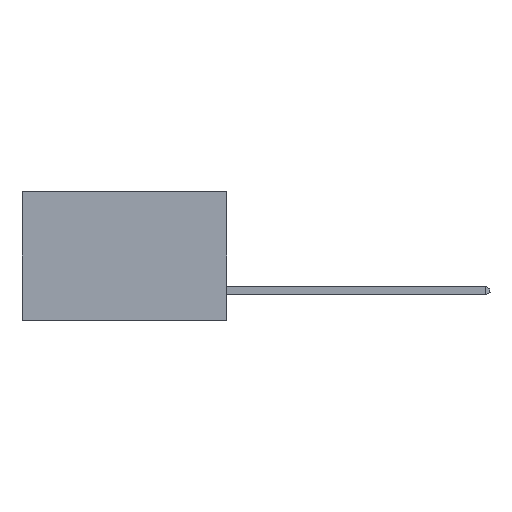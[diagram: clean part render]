
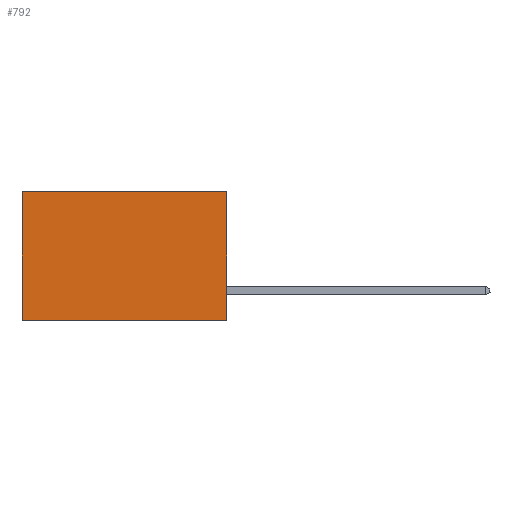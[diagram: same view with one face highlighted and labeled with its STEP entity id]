
A CAD part, left-side view. The second image highlights one B-rep face of the part: STEP entity #792.
In plain terms, the highlighted planar face has unit normal (-1, 0, 0).
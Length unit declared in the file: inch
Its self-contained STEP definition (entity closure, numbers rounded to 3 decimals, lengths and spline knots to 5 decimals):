
#745 = EDGE_CURVE ( 'NONE', #2251, #3498, #1872, .T. ) ;
#792 = ADVANCED_FACE ( 'NONE', ( #8173 ), #7313, .F. ) ;
#811 = VERTEX_POINT ( 'NONE', #3676 ) ;
#1142 = DIRECTION ( 'NONE',  ( 0., 0., -1. ) ) ;
#1163 = CARTESIAN_POINT ( 'NONE',  ( 0.277, 0., -0.37 ) ) ;
#1389 = LINE ( 'NONE', #1163, #8323 ) ;
#1849 = CARTESIAN_POINT ( 'NONE',  ( 0.277, 0., 0. ) ) ;
#1872 = LINE ( 'NONE', #6488, #7345 ) ;
#2251 = VERTEX_POINT ( 'NONE', #4747 ) ;
#2372 = DIRECTION ( 'NONE',  ( 0., 0., -1. ) ) ;
#3368 = DIRECTION ( 'NONE',  ( 0., 1., 0. ) ) ;
#3384 = CARTESIAN_POINT ( 'NONE',  ( 0.277, 0., -0.37 ) ) ;
#3392 = CARTESIAN_POINT ( 'NONE',  ( 0.277, 0., -0.37 ) ) ;
#3498 = VERTEX_POINT ( 'NONE', #4994 ) ;
#3511 = VECTOR ( 'NONE', #3368, 39.37008 ) ;
#3652 = ORIENTED_EDGE ( 'NONE', *, *, #745, .T. ) ;
#3676 = CARTESIAN_POINT ( 'NONE',  ( 0.277, 0., -0.37 ) ) ;
#3836 = EDGE_CURVE ( 'NONE', #811, #3498, #8687, .T. ) ;
#3866 = ORIENTED_EDGE ( 'NONE', *, *, #5896, .T. ) ;
#4086 = AXIS2_PLACEMENT_3D ( 'NONE', #3384, #6368, #6469 ) ;
#4171 = EDGE_CURVE ( 'NONE', #6514, #811, #1389, .T. ) ;
#4243 = EDGE_LOOP ( 'NONE', ( #3652, #5565, #7251, #3866 ) ) ;
#4747 = CARTESIAN_POINT ( 'NONE',  ( 0.277, 0.59, 0. ) ) ;
#4994 = CARTESIAN_POINT ( 'NONE',  ( 0.277, 0.59, -0.37 ) ) ;
#5565 = ORIENTED_EDGE ( 'NONE', *, *, #3836, .F. ) ;
#5896 = EDGE_CURVE ( 'NONE', #6514, #2251, #7583, .T. ) ;
#5906 = VECTOR ( 'NONE', #7559, 39.37008 ) ;
#6368 = DIRECTION ( 'NONE',  ( 1., 0., 0. ) ) ;
#6469 = DIRECTION ( 'NONE',  ( 0., 0., -1. ) ) ;
#6488 = CARTESIAN_POINT ( 'NONE',  ( 0.277, 0.59, -0.37 ) ) ;
#6514 = VERTEX_POINT ( 'NONE', #1849 ) ;
#6945 = CARTESIAN_POINT ( 'NONE',  ( 0.277, 0., 0. ) ) ;
#7251 = ORIENTED_EDGE ( 'NONE', *, *, #4171, .F. ) ;
#7313 = PLANE ( 'NONE',  #4086 ) ;
#7345 = VECTOR ( 'NONE', #2372, 39.37008 ) ;
#7559 = DIRECTION ( 'NONE',  ( 0., 1., 0. ) ) ;
#7583 = LINE ( 'NONE', #6945, #5906 ) ;
#8173 = FACE_OUTER_BOUND ( 'NONE', #4243, .T. ) ;
#8323 = VECTOR ( 'NONE', #1142, 39.37008 ) ;
#8687 = LINE ( 'NONE', #3392, #3511 ) ;
